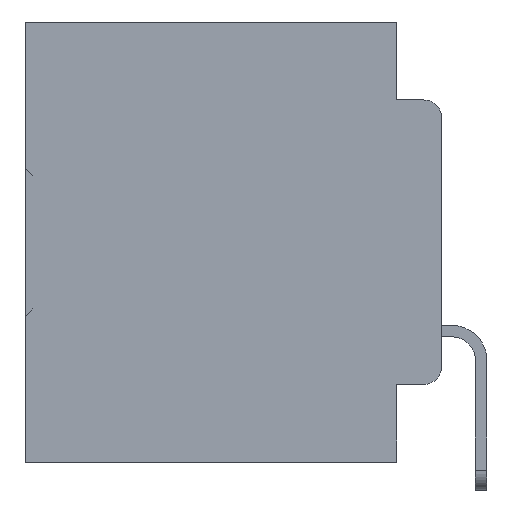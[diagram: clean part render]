
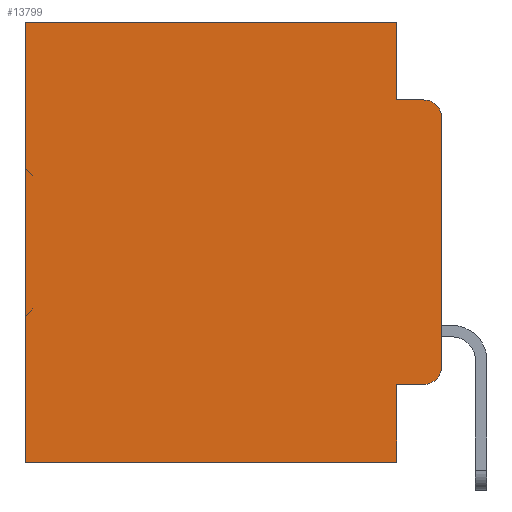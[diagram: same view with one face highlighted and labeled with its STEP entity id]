
A CAD part, left-side view. The second image highlights one B-rep face of the part: STEP entity #13799.
In plain terms, the highlighted planar face has unit normal (-1, 0, 0).
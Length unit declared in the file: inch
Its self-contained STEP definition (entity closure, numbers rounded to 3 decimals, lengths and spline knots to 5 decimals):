
#866 = VECTOR ( 'NONE', #19401, 39.37008 ) ;
#1167 = EDGE_CURVE ( 'NONE', #23316, #24999, #6964, .T. ) ;
#1469 = CARTESIAN_POINT ( 'NONE',  ( 0.298, 0.02, -0.1085 ) ) ;
#1523 = ORIENTED_EDGE ( 'NONE', *, *, #7430, .T. ) ;
#1690 = EDGE_LOOP ( 'NONE', ( #10445, #29011, #13462, #30882, #5743, #1523, #13610, #31261, #33047, #29298 ) ) ;
#1801 = LINE ( 'NONE', #19145, #23628 ) ;
#1878 = CARTESIAN_POINT ( 'NONE',  ( 0.298, 0.051, 0. ) ) ;
#1885 = LINE ( 'NONE', #36357, #866 ) ;
#2502 = VERTEX_POINT ( 'NONE', #10469 ) ;
#2679 = CARTESIAN_POINT ( 'NONE',  ( 0.298, 0.02, -0.0885 ) ) ;
#2785 = VECTOR ( 'NONE', #37597, 39.37008 ) ;
#3322 = EDGE_CURVE ( 'NONE', #34336, #23316, #1885, .T. ) ;
#3417 = AXIS2_PLACEMENT_3D ( 'NONE', #1469, #22315, #4664 ) ;
#3682 = VERTEX_POINT ( 'NONE', #8634 ) ;
#3789 = LINE ( 'NONE', #20659, #2785 ) ;
#4664 = DIRECTION ( 'NONE',  ( 0., 0., -1. ) ) ;
#4913 = DIRECTION ( 'NONE',  ( -1., 0., 0. ) ) ;
#5343 = LINE ( 'NONE', #33123, #12396 ) ;
#5389 = CARTESIAN_POINT ( 'NONE',  ( 0.298, 0.02, -0.4115 ) ) ;
#5396 = EDGE_CURVE ( 'NONE', #34336, #2502, #27926, .T. ) ;
#5611 = LINE ( 'NONE', #32419, #34543 ) ;
#5743 = ORIENTED_EDGE ( 'NONE', *, *, #20274, .T. ) ;
#5918 = DIRECTION ( 'NONE',  ( 1., 0., 0. ) ) ;
#6818 = FACE_OUTER_BOUND ( 'NONE', #1690, .T. ) ;
#6964 = CIRCLE ( 'NONE', #24431, 0.02 ) ;
#7430 = EDGE_CURVE ( 'NONE', #15515, #3682, #3789, .T. ) ;
#8352 = CARTESIAN_POINT ( 'NONE',  ( 0.298, 0.473, 0. ) ) ;
#8634 = CARTESIAN_POINT ( 'NONE',  ( 0.298, 0.473, -0.5 ) ) ;
#9450 = EDGE_CURVE ( 'NONE', #24547, #24648, #5611, .T. ) ;
#10445 = ORIENTED_EDGE ( 'NONE', *, *, #25018, .F. ) ;
#10469 = CARTESIAN_POINT ( 'NONE',  ( 0.298, 0.051, -0.5 ) ) ;
#12390 = DIRECTION ( 'NONE',  ( 0., 0., -1. ) ) ;
#12396 = VECTOR ( 'NONE', #35976, 39.37008 ) ;
#13020 = CARTESIAN_POINT ( 'NONE',  ( 0.298, 0., 0. ) ) ;
#13270 = CARTESIAN_POINT ( 'NONE',  ( 0.298, 0., -0.3915 ) ) ;
#13417 = EDGE_CURVE ( 'NONE', #24648, #18806, #5343, .T. ) ;
#13462 = ORIENTED_EDGE ( 'NONE', *, *, #13417, .F. ) ;
#13610 = ORIENTED_EDGE ( 'NONE', *, *, #13916, .F. ) ;
#13799 = ADVANCED_FACE ( 'NONE', ( #6818 ), #14741, .F. ) ;
#13916 = EDGE_CURVE ( 'NONE', #2502, #3682, #33016, .T. ) ;
#14741 = PLANE ( 'NONE',  #29422 ) ;
#15376 = EDGE_CURVE ( 'NONE', #33219, #18806, #36007, .T. ) ;
#15515 = VERTEX_POINT ( 'NONE', #8352 ) ;
#16092 = DIRECTION ( 'NONE',  ( 0., 1., 0. ) ) ;
#18806 = VERTEX_POINT ( 'NONE', #2679 ) ;
#19145 = CARTESIAN_POINT ( 'NONE',  ( 0.298, 0., 0. ) ) ;
#19401 = DIRECTION ( 'NONE',  ( 0., -1., 0. ) ) ;
#19471 = DIRECTION ( 'NONE',  ( 0., 0., -1. ) ) ;
#20260 = CARTESIAN_POINT ( 'NONE',  ( 0.298, 0.051, -0.4115 ) ) ;
#20274 = EDGE_CURVE ( 'NONE', #24547, #15515, #34092, .T. ) ;
#20395 = VECTOR ( 'NONE', #19471, 39.37008 ) ;
#20658 = CARTESIAN_POINT ( 'NONE',  ( 0.298, 0.02, -0.3915 ) ) ;
#20659 = CARTESIAN_POINT ( 'NONE',  ( 0.298, 0.473, 0. ) ) ;
#22315 = DIRECTION ( 'NONE',  ( -1., 0., 0. ) ) ;
#23316 = VERTEX_POINT ( 'NONE', #5389 ) ;
#23628 = VECTOR ( 'NONE', #33265, 39.37008 ) ;
#24085 = DIRECTION ( 'NONE',  ( 0., 1., 0. ) ) ;
#24431 = AXIS2_PLACEMENT_3D ( 'NONE', #20658, #4913, #32033 ) ;
#24547 = VERTEX_POINT ( 'NONE', #1878 ) ;
#24639 = VECTOR ( 'NONE', #24085, 39.37008 ) ;
#24648 = VERTEX_POINT ( 'NONE', #25867 ) ;
#24999 = VERTEX_POINT ( 'NONE', #13270 ) ;
#25018 = EDGE_CURVE ( 'NONE', #33219, #24999, #1801, .T. ) ;
#25867 = CARTESIAN_POINT ( 'NONE',  ( 0.298, 0.051, -0.0885 ) ) ;
#26291 = DIRECTION ( 'NONE',  ( 0., 0., -1. ) ) ;
#26573 = VECTOR ( 'NONE', #16092, 39.37008 ) ;
#26780 = CARTESIAN_POINT ( 'NONE',  ( 0.298, 0., -0.5 ) ) ;
#27926 = LINE ( 'NONE', #33589, #20395 ) ;
#29011 = ORIENTED_EDGE ( 'NONE', *, *, #15376, .T. ) ;
#29298 = ORIENTED_EDGE ( 'NONE', *, *, #1167, .T. ) ;
#29422 = AXIS2_PLACEMENT_3D ( 'NONE', #34685, #5918, #26291 ) ;
#30185 = CARTESIAN_POINT ( 'NONE',  ( 0.298, 0., -0.1085 ) ) ;
#30882 = ORIENTED_EDGE ( 'NONE', *, *, #9450, .F. ) ;
#31261 = ORIENTED_EDGE ( 'NONE', *, *, #5396, .F. ) ;
#32033 = DIRECTION ( 'NONE',  ( 0., 0., -1. ) ) ;
#32419 = CARTESIAN_POINT ( 'NONE',  ( 0.298, 0.051, 0. ) ) ;
#33016 = LINE ( 'NONE', #26780, #24639 ) ;
#33047 = ORIENTED_EDGE ( 'NONE', *, *, #3322, .T. ) ;
#33123 = CARTESIAN_POINT ( 'NONE',  ( 0.298, 0.051, -0.0885 ) ) ;
#33219 = VERTEX_POINT ( 'NONE', #30185 ) ;
#33265 = DIRECTION ( 'NONE',  ( 0., 0., -1. ) ) ;
#33589 = CARTESIAN_POINT ( 'NONE',  ( 0.298, 0.051, 0. ) ) ;
#34092 = LINE ( 'NONE', #13020, #26573 ) ;
#34336 = VERTEX_POINT ( 'NONE', #20260 ) ;
#34543 = VECTOR ( 'NONE', #12390, 39.37008 ) ;
#34685 = CARTESIAN_POINT ( 'NONE',  ( 0.298, 0., 0. ) ) ;
#35976 = DIRECTION ( 'NONE',  ( 0., -1., 0. ) ) ;
#36007 = CIRCLE ( 'NONE', #3417, 0.02 ) ;
#36357 = CARTESIAN_POINT ( 'NONE',  ( 0.298, 0.051, -0.4115 ) ) ;
#37597 = DIRECTION ( 'NONE',  ( 0., 0., -1. ) ) ;
